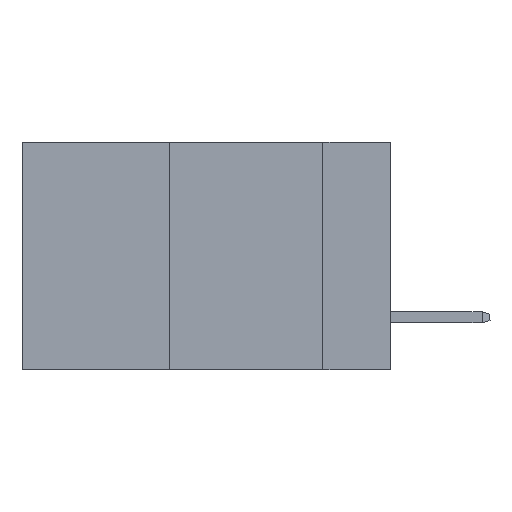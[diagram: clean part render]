
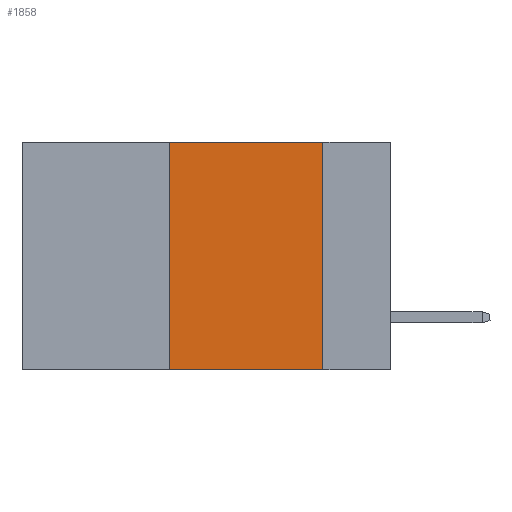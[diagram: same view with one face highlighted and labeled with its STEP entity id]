
A CAD part, left-side view. The second image highlights one B-rep face of the part: STEP entity #1858.
In plain terms, the highlighted planar face has unit normal (-1, 0, 0).
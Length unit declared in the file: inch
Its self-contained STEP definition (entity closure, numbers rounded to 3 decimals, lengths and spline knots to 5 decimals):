
#209 = DIRECTION ( 'NONE',  ( 0., 0., -1. ) ) ;
#493 = CARTESIAN_POINT ( 'NONE',  ( 0., 0.6, 0. ) ) ;
#566 = EDGE_LOOP ( 'NONE', ( #4537, #4690, #4716, #5036 ) ) ;
#591 = CARTESIAN_POINT ( 'NONE',  ( 0., 0.11, 0. ) ) ;
#950 = CARTESIAN_POINT ( 'NONE',  ( 0., 0.11, 0. ) ) ;
#1033 = LINE ( 'NONE', #950, #6599 ) ;
#1151 = DIRECTION ( 'NONE',  ( 0., 0., -1. ) ) ;
#1850 = CARTESIAN_POINT ( 'NONE',  ( 0., 0.36, -0.37 ) ) ;
#1858 = ADVANCED_FACE ( 'NONE', ( #7235 ), #2635, .F. ) ;
#1887 = CARTESIAN_POINT ( 'NONE',  ( 0., 0.36, 0. ) ) ;
#2563 = CARTESIAN_POINT ( 'NONE',  ( 0., 0.11, -0.37 ) ) ;
#2635 = PLANE ( 'NONE',  #11371 ) ;
#2661 = VECTOR ( 'NONE', #12544, 39.37008 ) ;
#2858 = VECTOR ( 'NONE', #8147, 39.37008 ) ;
#3178 = LINE ( 'NONE', #8090, #2858 ) ;
#3299 = EDGE_CURVE ( 'NONE', #12663, #8569, #1033, .T. ) ;
#3341 = EDGE_CURVE ( 'NONE', #8334, #12663, #3178, .T. ) ;
#4537 = ORIENTED_EDGE ( 'NONE', *, *, #3299, .F. ) ;
#4690 = ORIENTED_EDGE ( 'NONE', *, *, #3341, .F. ) ;
#4693 = CARTESIAN_POINT ( 'NONE',  ( 0., 0.36, 0. ) ) ;
#4716 = ORIENTED_EDGE ( 'NONE', *, *, #6765, .F. ) ;
#5036 = ORIENTED_EDGE ( 'NONE', *, *, #7330, .T. ) ;
#6599 = VECTOR ( 'NONE', #1151, 39.37008 ) ;
#6726 = VECTOR ( 'NONE', #9927, 39.37008 ) ;
#6765 = EDGE_CURVE ( 'NONE', #10346, #8334, #11833, .T. ) ;
#6920 = DIRECTION ( 'NONE',  ( 1., 0., 0. ) ) ;
#7235 = FACE_OUTER_BOUND ( 'NONE', #566, .T. ) ;
#7330 = EDGE_CURVE ( 'NONE', #10346, #8569, #8057, .T. ) ;
#8057 = LINE ( 'NONE', #10106, #2661 ) ;
#8090 = CARTESIAN_POINT ( 'NONE',  ( 0., 0.6, 0. ) ) ;
#8147 = DIRECTION ( 'NONE',  ( 0., -1., 0. ) ) ;
#8334 = VERTEX_POINT ( 'NONE', #4693 ) ;
#8569 = VERTEX_POINT ( 'NONE', #2563 ) ;
#9927 = DIRECTION ( 'NONE',  ( 0., 0., 1. ) ) ;
#10106 = CARTESIAN_POINT ( 'NONE',  ( 0., 0.6, -0.37 ) ) ;
#10346 = VERTEX_POINT ( 'NONE', #1850 ) ;
#11371 = AXIS2_PLACEMENT_3D ( 'NONE', #493, #6920, #209 ) ;
#11833 = LINE ( 'NONE', #1887, #6726 ) ;
#12544 = DIRECTION ( 'NONE',  ( 0., -1., 0. ) ) ;
#12663 = VERTEX_POINT ( 'NONE', #591 ) ;
